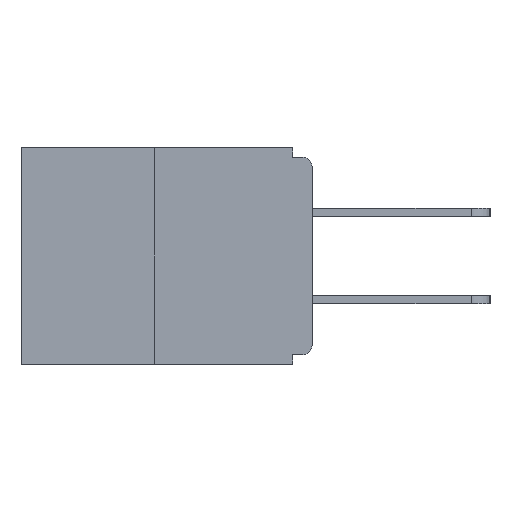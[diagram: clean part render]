
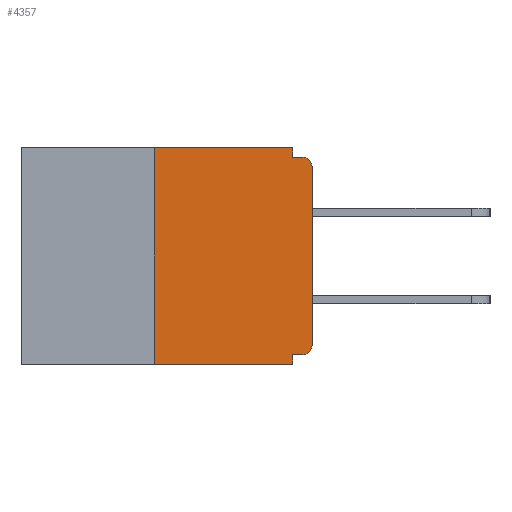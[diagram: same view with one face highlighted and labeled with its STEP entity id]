
A CAD part, left-side view. The second image highlights one B-rep face of the part: STEP entity #4357.
In plain terms, the highlighted planar face has unit normal (-1, 0, 0).
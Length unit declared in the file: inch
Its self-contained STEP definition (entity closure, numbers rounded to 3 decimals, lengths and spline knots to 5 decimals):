
#467 = PLANE ( 'NONE',  #10341 ) ;
#699 = VECTOR ( 'NONE', #11772, 39.37008 ) ;
#707 = CARTESIAN_POINT ( 'NONE',  ( 0., 0.25, -0.343 ) ) ;
#850 = LINE ( 'NONE', #16689, #6245 ) ;
#886 = VERTEX_POINT ( 'NONE', #6387 ) ;
#1051 = LINE ( 'NONE', #10294, #10368 ) ;
#1421 = EDGE_CURVE ( 'NONE', #886, #6970, #8871, .T. ) ;
#1589 = VERTEX_POINT ( 'NONE', #17005 ) ;
#1634 = DIRECTION ( 'NONE',  ( 0., 0., -1. ) ) ;
#1820 = VECTOR ( 'NONE', #15923, 39.37008 ) ;
#1947 = DIRECTION ( 'NONE',  ( 0., 0., -1. ) ) ;
#2028 = LINE ( 'NONE', #6180, #9785 ) ;
#2052 = VECTOR ( 'NONE', #1947, 39.37008 ) ;
#2334 = AXIS2_PLACEMENT_3D ( 'NONE', #13383, #6812, #1634 ) ;
#2367 = LINE ( 'NONE', #2761, #699 ) ;
#2645 = CARTESIAN_POINT ( 'NONE',  ( 0., 0., -0.03 ) ) ;
#2683 = CARTESIAN_POINT ( 'NONE',  ( 0., 0.46, -0.343 ) ) ;
#2761 = CARTESIAN_POINT ( 'NONE',  ( 0., 0.25, 0. ) ) ;
#2937 = VERTEX_POINT ( 'NONE', #11809 ) ;
#3245 = LINE ( 'NONE', #11477, #7171 ) ;
#3273 = EDGE_CURVE ( 'NONE', #10530, #9434, #2367, .T. ) ;
#3699 = VECTOR ( 'NONE', #7960, 39.37008 ) ;
#4008 = DIRECTION ( 'NONE',  ( -1., 0., 0. ) ) ;
#4357 = ADVANCED_FACE ( 'NONE', ( #5813 ), #467, .F. ) ;
#4426 = DIRECTION ( 'NONE',  ( 1., 0., 0. ) ) ;
#4487 = ORIENTED_EDGE ( 'NONE', *, *, #13440, .T. ) ;
#4778 = DIRECTION ( 'NONE',  ( 0., 1., 0. ) ) ;
#5683 = EDGE_CURVE ( 'NONE', #9434, #9454, #3245, .T. ) ;
#5786 = VERTEX_POINT ( 'NONE', #11818 ) ;
#5813 = FACE_OUTER_BOUND ( 'NONE', #10801, .T. ) ;
#6180 = CARTESIAN_POINT ( 'NONE',  ( 0., 0., -0.328 ) ) ;
#6245 = VECTOR ( 'NONE', #10112, 39.37008 ) ;
#6387 = CARTESIAN_POINT ( 'NONE',  ( 0., 0.031, -0.328 ) ) ;
#6812 = DIRECTION ( 'NONE',  ( -1., 0., 0. ) ) ;
#6970 = VERTEX_POINT ( 'NONE', #16442 ) ;
#7136 = DIRECTION ( 'NONE',  ( 0., -1., 0. ) ) ;
#7171 = VECTOR ( 'NONE', #7136, 39.37008 ) ;
#7485 = VERTEX_POINT ( 'NONE', #2645 ) ;
#7960 = DIRECTION ( 'NONE',  ( 0., -1., 0. ) ) ;
#8219 = ORIENTED_EDGE ( 'NONE', *, *, #3273, .F. ) ;
#8295 = CARTESIAN_POINT ( 'NONE',  ( 0., 0., 0. ) ) ;
#8597 = ORIENTED_EDGE ( 'NONE', *, *, #5683, .F. ) ;
#8871 = LINE ( 'NONE', #12573, #2052 ) ;
#8881 = CARTESIAN_POINT ( 'NONE',  ( 0., 0.015, -0.015 ) ) ;
#9087 = EDGE_CURVE ( 'NONE', #5786, #2937, #15848, .T. ) ;
#9195 = CARTESIAN_POINT ( 'NONE',  ( 0., 0.015, -0.313 ) ) ;
#9434 = VERTEX_POINT ( 'NONE', #10000 ) ;
#9454 = VERTEX_POINT ( 'NONE', #9666 ) ;
#9457 = DIRECTION ( 'NONE',  ( 0., 0., -1. ) ) ;
#9666 = CARTESIAN_POINT ( 'NONE',  ( 0., 0.031, 0. ) ) ;
#9785 = VECTOR ( 'NONE', #4778, 39.37008 ) ;
#9891 = ORIENTED_EDGE ( 'NONE', *, *, #9087, .T. ) ;
#9921 = ORIENTED_EDGE ( 'NONE', *, *, #15358, .F. ) ;
#10000 = CARTESIAN_POINT ( 'NONE',  ( 0., 0.25, 0. ) ) ;
#10076 = EDGE_CURVE ( 'NONE', #5786, #886, #2028, .T. ) ;
#10112 = DIRECTION ( 'NONE',  ( 0., 0., -1. ) ) ;
#10294 = CARTESIAN_POINT ( 'NONE',  ( 0., 0., -0.015 ) ) ;
#10341 = AXIS2_PLACEMENT_3D ( 'NONE', #16310, #4426, #9457 ) ;
#10368 = VECTOR ( 'NONE', #15565, 39.37008 ) ;
#10530 = VERTEX_POINT ( 'NONE', #707 ) ;
#10616 = ORIENTED_EDGE ( 'NONE', *, *, #11053, .F. ) ;
#10767 = ORIENTED_EDGE ( 'NONE', *, *, #11142, .T. ) ;
#10801 = EDGE_LOOP ( 'NONE', ( #8597, #8219, #4487, #11411, #13171, #9891, #10767, #16550, #10616, #9921 ) ) ;
#11053 = EDGE_CURVE ( 'NONE', #1589, #13302, #1051, .T. ) ;
#11142 = EDGE_CURVE ( 'NONE', #2937, #7485, #14675, .T. ) ;
#11411 = ORIENTED_EDGE ( 'NONE', *, *, #1421, .F. ) ;
#11477 = CARTESIAN_POINT ( 'NONE',  ( 0., 0.46, 0. ) ) ;
#11772 = DIRECTION ( 'NONE',  ( 0., 0., 1. ) ) ;
#11807 = DIRECTION ( 'NONE',  ( 0., 0., -1. ) ) ;
#11809 = CARTESIAN_POINT ( 'NONE',  ( 0., 0., -0.313 ) ) ;
#11818 = CARTESIAN_POINT ( 'NONE',  ( 0., 0.015, -0.328 ) ) ;
#12573 = CARTESIAN_POINT ( 'NONE',  ( 0., 0.031, -0.343 ) ) ;
#13171 = ORIENTED_EDGE ( 'NONE', *, *, #10076, .F. ) ;
#13302 = VERTEX_POINT ( 'NONE', #8881 ) ;
#13383 = CARTESIAN_POINT ( 'NONE',  ( 0., 0.015, -0.03 ) ) ;
#13440 = EDGE_CURVE ( 'NONE', #10530, #6970, #14522, .T. ) ;
#13444 = EDGE_CURVE ( 'NONE', #7485, #13302, #15056, .T. ) ;
#14522 = LINE ( 'NONE', #2683, #3699 ) ;
#14675 = LINE ( 'NONE', #8295, #1820 ) ;
#15056 = CIRCLE ( 'NONE', #2334, 0.015 ) ;
#15358 = EDGE_CURVE ( 'NONE', #9454, #1589, #850, .T. ) ;
#15565 = DIRECTION ( 'NONE',  ( 0., -1., 0. ) ) ;
#15848 = CIRCLE ( 'NONE', #15898, 0.015 ) ;
#15898 = AXIS2_PLACEMENT_3D ( 'NONE', #9195, #4008, #11807 ) ;
#15923 = DIRECTION ( 'NONE',  ( 0., 0., 1. ) ) ;
#16310 = CARTESIAN_POINT ( 'NONE',  ( 0., 0.46, 0. ) ) ;
#16442 = CARTESIAN_POINT ( 'NONE',  ( 0., 0.031, -0.343 ) ) ;
#16550 = ORIENTED_EDGE ( 'NONE', *, *, #13444, .T. ) ;
#16689 = CARTESIAN_POINT ( 'NONE',  ( 0., 0.031, 0. ) ) ;
#17005 = CARTESIAN_POINT ( 'NONE',  ( 0., 0.031, -0.015 ) ) ;
